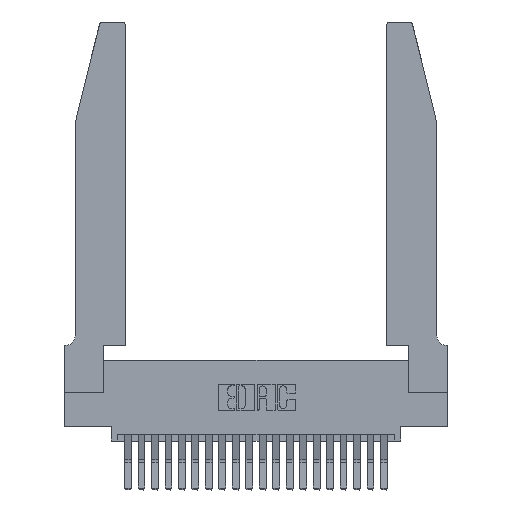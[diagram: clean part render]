
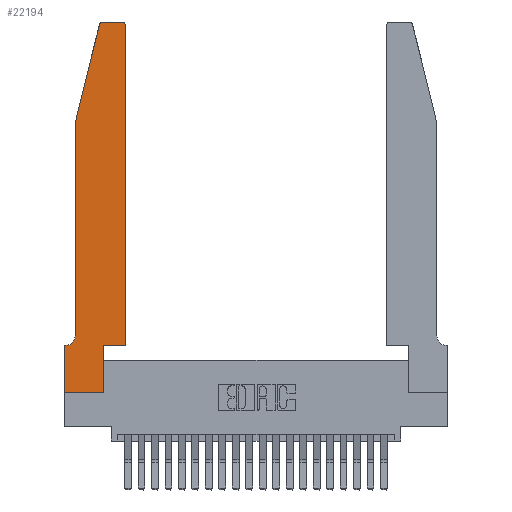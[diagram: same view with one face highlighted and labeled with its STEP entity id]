
A CAD part, top view. The second image highlights one B-rep face of the part: STEP entity #22194.
In plain terms, the highlighted planar face has unit normal (0, 0, 1).
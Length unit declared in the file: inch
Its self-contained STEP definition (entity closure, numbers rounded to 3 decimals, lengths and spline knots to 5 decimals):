
#138 = AXIS2_PLACEMENT_3D ( 'NONE', #11894, #770, #13704 ) ;
#448 = CARTESIAN_POINT ( 'NONE',  ( 0.2865, 0.35, 0.37 ) ) ;
#630 = ORIENTED_EDGE ( 'NONE', *, *, #18872, .T. ) ;
#770 = DIRECTION ( 'NONE',  ( 0., 0., 1. ) ) ;
#1376 = CARTESIAN_POINT ( 'NONE',  ( 0.0755, 0.35, 0.37 ) ) ;
#1656 = DIRECTION ( 'NONE',  ( 0., -1., 0. ) ) ;
#1904 = CARTESIAN_POINT ( 'NONE',  ( 0.4505, 2.72, 0.37 ) ) ;
#2094 = CIRCLE ( 'NONE', #4319, 0.07 ) ;
#2135 = EDGE_CURVE ( 'NONE', #17840, #15114, #4846, .T. ) ;
#2156 = ORIENTED_EDGE ( 'NONE', *, *, #10663, .T. ) ;
#2756 = ORIENTED_EDGE ( 'NONE', *, *, #23004, .T. ) ;
#2971 = CARTESIAN_POINT ( 'NONE',  ( 0.4505, 0.35, 0.37 ) ) ;
#3167 = CARTESIAN_POINT ( 'NONE',  ( 0.0755, 2., 0.37 ) ) ;
#3251 = VERTEX_POINT ( 'NONE', #1904 ) ;
#3329 = DIRECTION ( 'NONE',  ( 0., -1., 0. ) ) ;
#3637 = ORIENTED_EDGE ( 'NONE', *, *, #16168, .T. ) ;
#4108 = VERTEX_POINT ( 'NONE', #19841 ) ;
#4272 = FACE_OUTER_BOUND ( 'NONE', #15146, .T. ) ;
#4319 = AXIS2_PLACEMENT_3D ( 'NONE', #19987, #9094, #21742 ) ;
#4457 = CARTESIAN_POINT ( 'NONE',  ( 0.0755, 2., 0.37 ) ) ;
#4506 = ORIENTED_EDGE ( 'NONE', *, *, #13610, .T. ) ;
#4570 = CARTESIAN_POINT ( 'NONE',  ( 0.4505, 0.35, 0.37 ) ) ;
#4778 = ORIENTED_EDGE ( 'NONE', *, *, #6883, .T. ) ;
#4846 = LINE ( 'NONE', #18199, #23498 ) ;
#5357 = LINE ( 'NONE', #3167, #14490 ) ;
#5690 = LINE ( 'NONE', #12699, #10038 ) ;
#5838 = CARTESIAN_POINT ( 'NONE',  ( 0., 0., 0.37 ) ) ;
#5904 = ORIENTED_EDGE ( 'NONE', *, *, #10750, .T. ) ;
#6024 = VERTEX_POINT ( 'NONE', #7162 ) ;
#6028 = CIRCLE ( 'NONE', #6436, 0.03 ) ;
#6300 = DIRECTION ( 'NONE',  ( 1., 0., 0. ) ) ;
#6436 = AXIS2_PLACEMENT_3D ( 'NONE', #20818, #9981, #22547 ) ;
#6731 = CARTESIAN_POINT ( 'NONE',  ( 0., 0.35, 0.37 ) ) ;
#6883 = EDGE_CURVE ( 'NONE', #6024, #17247, #9806, .T. ) ;
#6911 = DIRECTION ( 'NONE',  ( -1., 0., 0. ) ) ;
#7162 = CARTESIAN_POINT ( 'NONE',  ( 0.25487, 2.72718, 0.37 ) ) ;
#8063 = AXIS2_PLACEMENT_3D ( 'NONE', #6731, #8596, #21269 ) ;
#8518 = CARTESIAN_POINT ( 'NONE',  ( 0.2865, 0., 0.37 ) ) ;
#8596 = DIRECTION ( 'NONE',  ( 0., 0., 1. ) ) ;
#8750 = CARTESIAN_POINT ( 'NONE',  ( 0.0755, 0.42, 0.37 ) ) ;
#8770 = VECTOR ( 'NONE', #6911, 39.37008 ) ;
#9094 = DIRECTION ( 'NONE',  ( 0., 0., -1. ) ) ;
#9806 = LINE ( 'NONE', #14721, #23557 ) ;
#9981 = DIRECTION ( 'NONE',  ( 0., 0., 1. ) ) ;
#9985 = ORIENTED_EDGE ( 'NONE', *, *, #20384, .T. ) ;
#10038 = VECTOR ( 'NONE', #1656, 39.37008 ) ;
#10479 = CIRCLE ( 'NONE', #138, 0.03 ) ;
#10658 = VECTOR ( 'NONE', #6300, 39.37008 ) ;
#10663 = EDGE_CURVE ( 'NONE', #12964, #4108, #22573, .T. ) ;
#10750 = EDGE_CURVE ( 'NONE', #20561, #12964, #2094, .T. ) ;
#10801 = EDGE_CURVE ( 'NONE', #22160, #22614, #15000, .T. ) ;
#11203 = CARTESIAN_POINT ( 'NONE',  ( 0.4505, 0.35, 0.37 ) ) ;
#11233 = CARTESIAN_POINT ( 'NONE',  ( 0.0055, 0.35, 0.37 ) ) ;
#11894 = CARTESIAN_POINT ( 'NONE',  ( 0.4205, 2.72, 0.37 ) ) ;
#12391 = LINE ( 'NONE', #4570, #21429 ) ;
#12699 = CARTESIAN_POINT ( 'NONE',  ( 0., 0., 0.37 ) ) ;
#12964 = VERTEX_POINT ( 'NONE', #11233 ) ;
#13034 = DIRECTION ( 'NONE',  ( 1., 0., 0. ) ) ;
#13610 = EDGE_CURVE ( 'NONE', #22614, #18968, #21199, .T. ) ;
#13681 = DIRECTION ( 'NONE',  ( 0., 1., 0. ) ) ;
#13704 = DIRECTION ( 'NONE',  ( 1., 0., 0. ) ) ;
#13988 = PLANE ( 'NONE',  #8063 ) ;
#14435 = VECTOR ( 'NONE', #20133, 39.37008 ) ;
#14490 = VECTOR ( 'NONE', #3329, 39.37008 ) ;
#14721 = CARTESIAN_POINT ( 'NONE',  ( 0.0755, 2., 0.37 ) ) ;
#15000 = LINE ( 'NONE', #18320, #14435 ) ;
#15114 = VERTEX_POINT ( 'NONE', #17490 ) ;
#15146 = EDGE_LOOP ( 'NONE', ( #17048, #3637, #4778, #19913, #5904, #2156, #2756, #22086, #18491, #4506, #9985, #630 ) ) ;
#15840 = VECTOR ( 'NONE', #13034, 39.37008 ) ;
#16168 = EDGE_CURVE ( 'NONE', #15114, #6024, #6028, .T. ) ;
#17048 = ORIENTED_EDGE ( 'NONE', *, *, #2135, .T. ) ;
#17247 = VERTEX_POINT ( 'NONE', #4457 ) ;
#17490 = CARTESIAN_POINT ( 'NONE',  ( 0.284, 2.75, 0.37 ) ) ;
#17647 = VERTEX_POINT ( 'NONE', #5838 ) ;
#17670 = CARTESIAN_POINT ( 'NONE',  ( 0.4205, 2.75, 0.37 ) ) ;
#17840 = VERTEX_POINT ( 'NONE', #17670 ) ;
#18199 = CARTESIAN_POINT ( 'NONE',  ( 0.2605, 2.75, 0.37 ) ) ;
#18320 = CARTESIAN_POINT ( 'NONE',  ( 0.2865, 0.35, 0.37 ) ) ;
#18386 = DIRECTION ( 'NONE',  ( -0.239, -0.971, 0. ) ) ;
#18491 = ORIENTED_EDGE ( 'NONE', *, *, #10801, .T. ) ;
#18522 = EDGE_CURVE ( 'NONE', #17247, #20561, #5357, .T. ) ;
#18872 = EDGE_CURVE ( 'NONE', #3251, #17840, #10479, .T. ) ;
#18968 = VERTEX_POINT ( 'NONE', #2971 ) ;
#19067 = CARTESIAN_POINT ( 'NONE',  ( 0., 0., 0.37 ) ) ;
#19841 = CARTESIAN_POINT ( 'NONE',  ( 0., 0.35, 0.37 ) ) ;
#19913 = ORIENTED_EDGE ( 'NONE', *, *, #18522, .T. ) ;
#19987 = CARTESIAN_POINT ( 'NONE',  ( 0.0055, 0.42, 0.37 ) ) ;
#20133 = DIRECTION ( 'NONE',  ( 0., 1., 0. ) ) ;
#20301 = LINE ( 'NONE', #19067, #10658 ) ;
#20384 = EDGE_CURVE ( 'NONE', #18968, #3251, #12391, .T. ) ;
#20561 = VERTEX_POINT ( 'NONE', #8750 ) ;
#20653 = DIRECTION ( 'NONE',  ( -1., 0., 0. ) ) ;
#20818 = CARTESIAN_POINT ( 'NONE',  ( 0.284, 2.72, 0.37 ) ) ;
#20917 = EDGE_CURVE ( 'NONE', #17647, #22160, #20301, .T. ) ;
#21199 = LINE ( 'NONE', #11203, #15840 ) ;
#21269 = DIRECTION ( 'NONE',  ( 1., 0., 0. ) ) ;
#21429 = VECTOR ( 'NONE', #13681, 39.37008 ) ;
#21742 = DIRECTION ( 'NONE',  ( -1., 0., 0. ) ) ;
#22086 = ORIENTED_EDGE ( 'NONE', *, *, #20917, .T. ) ;
#22160 = VERTEX_POINT ( 'NONE', #8518 ) ;
#22194 = ADVANCED_FACE ( 'NONE', ( #4272 ), #13988, .T. ) ;
#22547 = DIRECTION ( 'NONE',  ( 1., 0., 0. ) ) ;
#22573 = LINE ( 'NONE', #1376, #8770 ) ;
#22614 = VERTEX_POINT ( 'NONE', #448 ) ;
#23004 = EDGE_CURVE ( 'NONE', #4108, #17647, #5690, .T. ) ;
#23498 = VECTOR ( 'NONE', #20653, 39.37008 ) ;
#23557 = VECTOR ( 'NONE', #18386, 39.37008 ) ;
